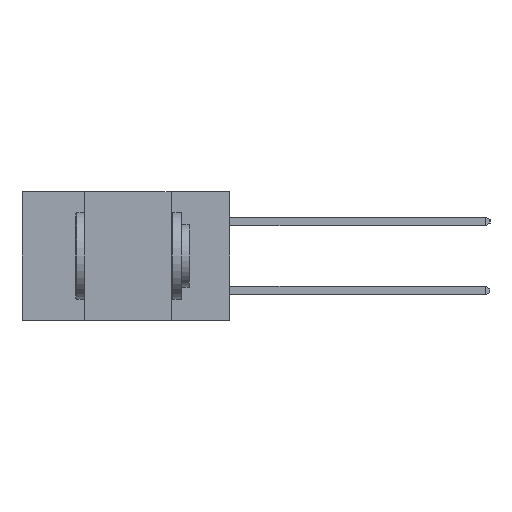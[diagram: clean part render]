
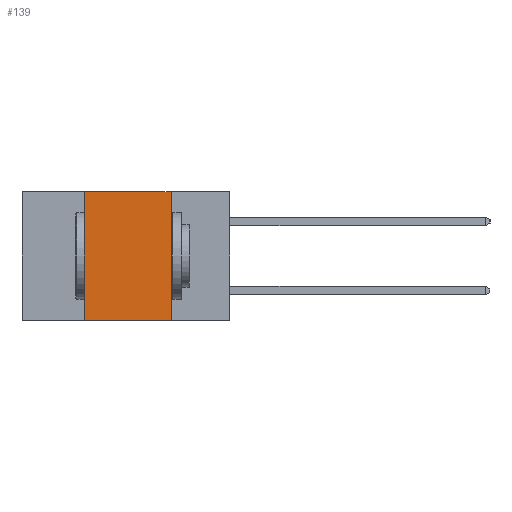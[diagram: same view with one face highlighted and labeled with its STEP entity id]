
A CAD part, left-side view. The second image highlights one B-rep face of the part: STEP entity #139.
In plain terms, the highlighted planar face has unit normal (-1, 0, 0).
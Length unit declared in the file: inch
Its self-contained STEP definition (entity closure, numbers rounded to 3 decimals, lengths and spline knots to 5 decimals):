
#21 = ORIENTED_EDGE ( 'NONE', *, *, #6185, .F. ) ;
#139 = ADVANCED_FACE ( 'NONE', ( #9331 ), #7140, .F. ) ;
#735 = EDGE_CURVE ( 'NONE', #2677, #6223, #12974, .T. ) ;
#1154 = DIRECTION ( 'NONE',  ( 0., 0., -1. ) ) ;
#1673 = CARTESIAN_POINT ( 'NONE',  ( 0., 0.42, 0. ) ) ;
#1888 = VECTOR ( 'NONE', #4495, 39.37008 ) ;
#2128 = CARTESIAN_POINT ( 'NONE',  ( 0., 0.17, -0.37 ) ) ;
#2664 = VECTOR ( 'NONE', #3370, 39.37008 ) ;
#2677 = VERTEX_POINT ( 'NONE', #4858 ) ;
#3072 = VERTEX_POINT ( 'NONE', #1673 ) ;
#3370 = DIRECTION ( 'NONE',  ( 0., -1., 0. ) ) ;
#3392 = VECTOR ( 'NONE', #3876, 39.37008 ) ;
#3403 = EDGE_CURVE ( 'NONE', #3072, #5333, #3703, .T. ) ;
#3703 = LINE ( 'NONE', #8866, #3392 ) ;
#3876 = DIRECTION ( 'NONE',  ( 0., -1., 0. ) ) ;
#4218 = CARTESIAN_POINT ( 'NONE',  ( 0., 0.6, -0.37 ) ) ;
#4228 = EDGE_CURVE ( 'NONE', #2677, #3072, #4603, .T. ) ;
#4368 = ORIENTED_EDGE ( 'NONE', *, *, #4228, .F. ) ;
#4495 = DIRECTION ( 'NONE',  ( 0., 0., 1. ) ) ;
#4603 = LINE ( 'NONE', #5792, #1888 ) ;
#4858 = CARTESIAN_POINT ( 'NONE',  ( 0., 0.42, -0.37 ) ) ;
#5333 = VERTEX_POINT ( 'NONE', #6587 ) ;
#5542 = CARTESIAN_POINT ( 'NONE',  ( 0., 0.17, 0. ) ) ;
#5792 = CARTESIAN_POINT ( 'NONE',  ( 0., 0.42, 0. ) ) ;
#6085 = AXIS2_PLACEMENT_3D ( 'NONE', #9689, #12239, #13136 ) ;
#6185 = EDGE_CURVE ( 'NONE', #5333, #6223, #8083, .T. ) ;
#6223 = VERTEX_POINT ( 'NONE', #2128 ) ;
#6587 = CARTESIAN_POINT ( 'NONE',  ( 0., 0.17, 0. ) ) ;
#7140 = PLANE ( 'NONE',  #6085 ) ;
#7761 = EDGE_LOOP ( 'NONE', ( #21, #11456, #4368, #12349 ) ) ;
#8083 = LINE ( 'NONE', #5542, #12978 ) ;
#8866 = CARTESIAN_POINT ( 'NONE',  ( 0., 0.6, 0. ) ) ;
#9331 = FACE_OUTER_BOUND ( 'NONE', #7761, .T. ) ;
#9689 = CARTESIAN_POINT ( 'NONE',  ( 0., 0.6, 0. ) ) ;
#11456 = ORIENTED_EDGE ( 'NONE', *, *, #3403, .F. ) ;
#12239 = DIRECTION ( 'NONE',  ( 1., 0., 0. ) ) ;
#12349 = ORIENTED_EDGE ( 'NONE', *, *, #735, .T. ) ;
#12974 = LINE ( 'NONE', #4218, #2664 ) ;
#12978 = VECTOR ( 'NONE', #1154, 39.37008 ) ;
#13136 = DIRECTION ( 'NONE',  ( 0., 0., -1. ) ) ;
